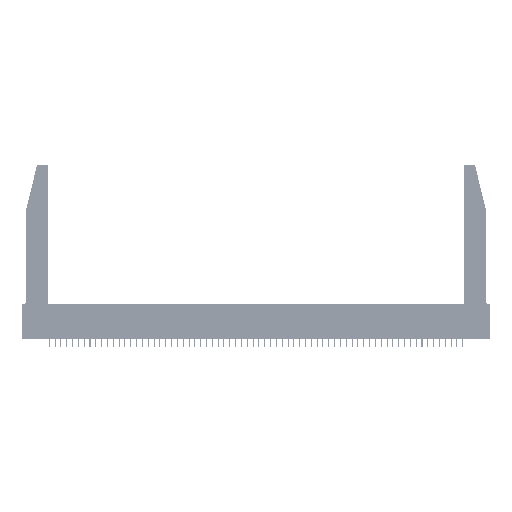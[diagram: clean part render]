
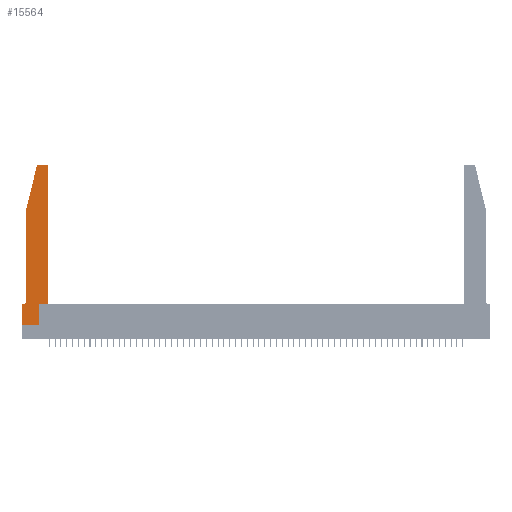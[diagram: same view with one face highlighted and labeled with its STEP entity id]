
A CAD part, top view. The second image highlights one B-rep face of the part: STEP entity #15564.
In plain terms, the highlighted planar face has unit normal (0, 0, 1).
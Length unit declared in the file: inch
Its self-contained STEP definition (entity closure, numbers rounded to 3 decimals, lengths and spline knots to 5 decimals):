
#433 = VECTOR ( 'NONE', #41303, 39.37008 ) ;
#551 = ORIENTED_EDGE ( 'NONE', *, *, #21528, .T. ) ;
#1624 = EDGE_CURVE ( 'NONE', #32058, #23800, #53477, .T. ) ;
#1963 = ORIENTED_EDGE ( 'NONE', *, *, #54328, .T. ) ;
#2936 = VECTOR ( 'NONE', #52569, 39.37008 ) ;
#3967 = ORIENTED_EDGE ( 'NONE', *, *, #13492, .T. ) ;
#5809 = DIRECTION ( 'NONE',  ( 0., -1., 0. ) ) ;
#6482 = CARTESIAN_POINT ( 'NONE',  ( 0.2865, 0., 0.37 ) ) ;
#6486 = CARTESIAN_POINT ( 'NONE',  ( 0.4505, 0.35, 0.37 ) ) ;
#7145 = AXIS2_PLACEMENT_3D ( 'NONE', #8463, #26193, #39527 ) ;
#7485 = VERTEX_POINT ( 'NONE', #40664 ) ;
#8364 = EDGE_CURVE ( 'NONE', #9404, #48864, #27980, .T. ) ;
#8463 = CARTESIAN_POINT ( 'NONE',  ( 0.4205, 2.72, 0.37 ) ) ;
#9404 = VERTEX_POINT ( 'NONE', #43665 ) ;
#9867 = VECTOR ( 'NONE', #5809, 39.37008 ) ;
#10137 = CARTESIAN_POINT ( 'NONE',  ( 0.2865, 0.35, 0.37 ) ) ;
#10265 = VECTOR ( 'NONE', #35237, 39.37008 ) ;
#10976 = CARTESIAN_POINT ( 'NONE',  ( 0.284, 2.72, 0.37 ) ) ;
#11841 = CARTESIAN_POINT ( 'NONE',  ( 0.4505, 0.35, 0.37 ) ) ;
#12476 = DIRECTION ( 'NONE',  ( 1., 0., 0. ) ) ;
#13271 = VERTEX_POINT ( 'NONE', #17739 ) ;
#13492 = EDGE_CURVE ( 'NONE', #46943, #21508, #41793, .T. ) ;
#13991 = CARTESIAN_POINT ( 'NONE',  ( 0.0755, 2., 0.37 ) ) ;
#14966 = DIRECTION ( 'NONE',  ( 1., 0., 0. ) ) ;
#15062 = CARTESIAN_POINT ( 'NONE',  ( 0.284, 2.75, 0.37 ) ) ;
#15564 = ADVANCED_FACE ( 'NONE', ( #19078 ), #36456, .T. ) ;
#16835 = VECTOR ( 'NONE', #53092, 39.37008 ) ;
#17126 = CIRCLE ( 'NONE', #37545, 0.07 ) ;
#17739 = CARTESIAN_POINT ( 'NONE',  ( 0., 0., 0.37 ) ) ;
#18007 = DIRECTION ( 'NONE',  ( -1., 0., 0. ) ) ;
#18300 = LINE ( 'NONE', #35694, #23059 ) ;
#19024 = CARTESIAN_POINT ( 'NONE',  ( 0.25487, 2.72718, 0.37 ) ) ;
#19078 = FACE_OUTER_BOUND ( 'NONE', #27872, .T. ) ;
#19580 = ORIENTED_EDGE ( 'NONE', *, *, #1624, .T. ) ;
#20002 = DIRECTION ( 'NONE',  ( 1., 0., 0. ) ) ;
#21508 = VERTEX_POINT ( 'NONE', #31654 ) ;
#21528 = EDGE_CURVE ( 'NONE', #36167, #46943, #57311, .T. ) ;
#22060 = ORIENTED_EDGE ( 'NONE', *, *, #41936, .T. ) ;
#23059 = VECTOR ( 'NONE', #18007, 39.37008 ) ;
#23178 = CIRCLE ( 'NONE', #35191, 0.03 ) ;
#23800 = VERTEX_POINT ( 'NONE', #53221 ) ;
#26193 = DIRECTION ( 'NONE',  ( 0., 0., 1. ) ) ;
#26425 = LINE ( 'NONE', #56565, #55729 ) ;
#26822 = EDGE_CURVE ( 'NONE', #21508, #39274, #17126, .T. ) ;
#27690 = AXIS2_PLACEMENT_3D ( 'NONE', #28619, #32113, #14966 ) ;
#27872 = EDGE_LOOP ( 'NONE', ( #30469, #1963, #551, #3967, #45755, #22060, #35063, #56746, #42180, #38162, #19580, #36635 ) ) ;
#27980 = LINE ( 'NONE', #36667, #46675 ) ;
#28619 = CARTESIAN_POINT ( 'NONE',  ( 0., 0.35, 0.37 ) ) ;
#28986 = DIRECTION ( 'NONE',  ( 1., 0., 0. ) ) ;
#29291 = CARTESIAN_POINT ( 'NONE',  ( 0.0055, 0.42, 0.37 ) ) ;
#29422 = CIRCLE ( 'NONE', #7145, 0.03 ) ;
#29575 = DIRECTION ( 'NONE',  ( 0., 0., -1. ) ) ;
#30469 = ORIENTED_EDGE ( 'NONE', *, *, #8364, .T. ) ;
#30549 = LINE ( 'NONE', #35173, #2936 ) ;
#31654 = CARTESIAN_POINT ( 'NONE',  ( 0.0755, 0.42, 0.37 ) ) ;
#32058 = VERTEX_POINT ( 'NONE', #6486 ) ;
#32113 = DIRECTION ( 'NONE',  ( 0., 0., 1. ) ) ;
#33362 = DIRECTION ( 'NONE',  ( -1., 0., 0. ) ) ;
#33625 = LINE ( 'NONE', #11841, #50517 ) ;
#35063 = ORIENTED_EDGE ( 'NONE', *, *, #46835, .T. ) ;
#35173 = CARTESIAN_POINT ( 'NONE',  ( 0., 0., 0.37 ) ) ;
#35191 = AXIS2_PLACEMENT_3D ( 'NONE', #10976, #46356, #20002 ) ;
#35237 = DIRECTION ( 'NONE',  ( 0., 1., 0. ) ) ;
#35413 = CARTESIAN_POINT ( 'NONE',  ( 0.0755, 2., 0.37 ) ) ;
#35694 = CARTESIAN_POINT ( 'NONE',  ( 0.0755, 0.35, 0.37 ) ) ;
#35784 = CARTESIAN_POINT ( 'NONE',  ( 0.4505, 0.35, 0.37 ) ) ;
#35816 = LINE ( 'NONE', #53210, #10265 ) ;
#36167 = VERTEX_POINT ( 'NONE', #19024 ) ;
#36330 = VERTEX_POINT ( 'NONE', #6482 ) ;
#36456 = PLANE ( 'NONE',  #27690 ) ;
#36575 = VERTEX_POINT ( 'NONE', #10137 ) ;
#36635 = ORIENTED_EDGE ( 'NONE', *, *, #38969, .T. ) ;
#36667 = CARTESIAN_POINT ( 'NONE',  ( 0.2605, 2.75, 0.37 ) ) ;
#36843 = EDGE_CURVE ( 'NONE', #36575, #32058, #33625, .T. ) ;
#36883 = CARTESIAN_POINT ( 'NONE',  ( 0.0055, 0.35, 0.37 ) ) ;
#37212 = DIRECTION ( 'NONE',  ( -1., 0., 0. ) ) ;
#37545 = AXIS2_PLACEMENT_3D ( 'NONE', #29291, #29575, #33362 ) ;
#38162 = ORIENTED_EDGE ( 'NONE', *, *, #36843, .T. ) ;
#38969 = EDGE_CURVE ( 'NONE', #23800, #9404, #29422, .T. ) ;
#39274 = VERTEX_POINT ( 'NONE', #36883 ) ;
#39527 = DIRECTION ( 'NONE',  ( 1., 0., 0. ) ) ;
#40664 = CARTESIAN_POINT ( 'NONE',  ( 0., 0.35, 0.37 ) ) ;
#41303 = DIRECTION ( 'NONE',  ( 0., 1., 0. ) ) ;
#41793 = LINE ( 'NONE', #45548, #9867 ) ;
#41936 = EDGE_CURVE ( 'NONE', #39274, #7485, #18300, .T. ) ;
#42180 = ORIENTED_EDGE ( 'NONE', *, *, #44980, .T. ) ;
#43665 = CARTESIAN_POINT ( 'NONE',  ( 0.4205, 2.75, 0.37 ) ) ;
#44980 = EDGE_CURVE ( 'NONE', #36330, #36575, #35816, .T. ) ;
#45548 = CARTESIAN_POINT ( 'NONE',  ( 0.0755, 2., 0.37 ) ) ;
#45755 = ORIENTED_EDGE ( 'NONE', *, *, #26822, .T. ) ;
#45905 = EDGE_CURVE ( 'NONE', #13271, #36330, #26425, .T. ) ;
#46356 = DIRECTION ( 'NONE',  ( 0., 0., 1. ) ) ;
#46675 = VECTOR ( 'NONE', #37212, 39.37008 ) ;
#46835 = EDGE_CURVE ( 'NONE', #7485, #13271, #30549, .T. ) ;
#46943 = VERTEX_POINT ( 'NONE', #13991 ) ;
#48864 = VERTEX_POINT ( 'NONE', #15062 ) ;
#50517 = VECTOR ( 'NONE', #28986, 39.37008 ) ;
#52569 = DIRECTION ( 'NONE',  ( 0., -1., 0. ) ) ;
#53092 = DIRECTION ( 'NONE',  ( -0.239, -0.971, 0. ) ) ;
#53210 = CARTESIAN_POINT ( 'NONE',  ( 0.2865, 0.35, 0.37 ) ) ;
#53221 = CARTESIAN_POINT ( 'NONE',  ( 0.4505, 2.72, 0.37 ) ) ;
#53477 = LINE ( 'NONE', #35784, #433 ) ;
#54328 = EDGE_CURVE ( 'NONE', #48864, #36167, #23178, .T. ) ;
#55729 = VECTOR ( 'NONE', #12476, 39.37008 ) ;
#56565 = CARTESIAN_POINT ( 'NONE',  ( 0., 0., 0.37 ) ) ;
#56746 = ORIENTED_EDGE ( 'NONE', *, *, #45905, .T. ) ;
#57311 = LINE ( 'NONE', #35413, #16835 ) ;
